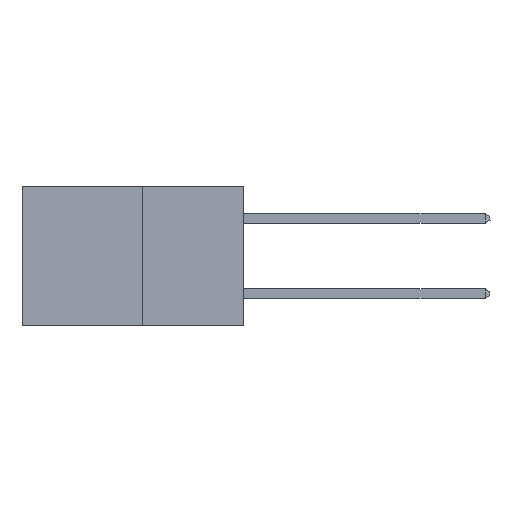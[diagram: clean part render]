
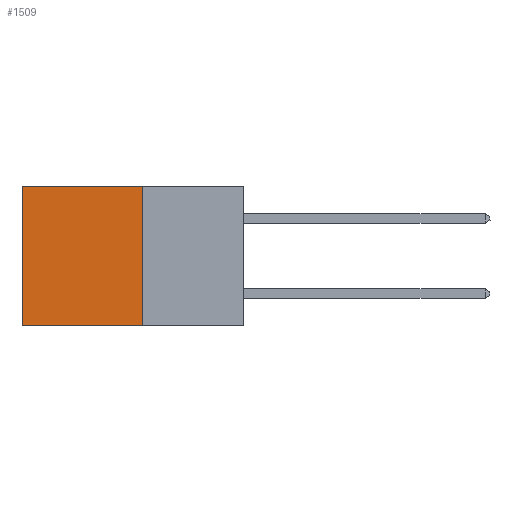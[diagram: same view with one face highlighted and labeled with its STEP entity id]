
A CAD part, left-side view. The second image highlights one B-rep face of the part: STEP entity #1509.
In plain terms, the highlighted planar face has unit normal (-1, 0, 0).
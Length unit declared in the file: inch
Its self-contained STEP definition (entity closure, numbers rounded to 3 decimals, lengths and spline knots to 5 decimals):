
#188 = ORIENTED_EDGE ( 'NONE', *, *, #4022, .T. ) ;
#232 = VERTEX_POINT ( 'NONE', #1717 ) ;
#594 = LINE ( 'NONE', #9998, #5398 ) ;
#685 = ORIENTED_EDGE ( 'NONE', *, *, #2946, .F. ) ;
#1406 = VERTEX_POINT ( 'NONE', #11083 ) ;
#1481 = AXIS2_PLACEMENT_3D ( 'NONE', #5484, #7393, #5969 ) ;
#1509 = ADVANCED_FACE ( 'NONE', ( #4404 ), #5711, .F. ) ;
#1717 = CARTESIAN_POINT ( 'NONE',  ( 0.277, 0.27, 0. ) ) ;
#2160 = EDGE_CURVE ( 'NONE', #1406, #3492, #8830, .T. ) ;
#2493 = EDGE_LOOP ( 'NONE', ( #188, #2841, #685, #4034 ) ) ;
#2841 = ORIENTED_EDGE ( 'NONE', *, *, #2160, .F. ) ;
#2946 = EDGE_CURVE ( 'NONE', #232, #1406, #10868, .T. ) ;
#3453 = VECTOR ( 'NONE', #9688, 39.37008 ) ;
#3492 = VERTEX_POINT ( 'NONE', #6788 ) ;
#4022 = EDGE_CURVE ( 'NONE', #5040, #3492, #594, .T. ) ;
#4034 = ORIENTED_EDGE ( 'NONE', *, *, #4761, .T. ) ;
#4404 = FACE_OUTER_BOUND ( 'NONE', #2493, .T. ) ;
#4761 = EDGE_CURVE ( 'NONE', #232, #5040, #9844, .T. ) ;
#5040 = VERTEX_POINT ( 'NONE', #11506 ) ;
#5154 = CARTESIAN_POINT ( 'NONE',  ( 0.277, 0.27, -0.37 ) ) ;
#5398 = VECTOR ( 'NONE', #9977, 39.37008 ) ;
#5484 = CARTESIAN_POINT ( 'NONE',  ( 0.277, 0.27, -0.37 ) ) ;
#5711 = PLANE ( 'NONE',  #1481 ) ;
#5969 = DIRECTION ( 'NONE',  ( 0., 0., -1. ) ) ;
#6788 = CARTESIAN_POINT ( 'NONE',  ( 0.277, 0.59, -0.37 ) ) ;
#7161 = DIRECTION ( 'NONE',  ( 0., 1., 0. ) ) ;
#7171 = CARTESIAN_POINT ( 'NONE',  ( 0.277, 0.27, 0. ) ) ;
#7393 = DIRECTION ( 'NONE',  ( 1., 0., 0. ) ) ;
#8791 = DIRECTION ( 'NONE',  ( 0., 0., -1. ) ) ;
#8806 = VECTOR ( 'NONE', #8791, 39.37008 ) ;
#8830 = LINE ( 'NONE', #5154, #3453 ) ;
#9688 = DIRECTION ( 'NONE',  ( 0., 1., 0. ) ) ;
#9844 = LINE ( 'NONE', #7171, #11463 ) ;
#9977 = DIRECTION ( 'NONE',  ( 0., 0., -1. ) ) ;
#9998 = CARTESIAN_POINT ( 'NONE',  ( 0.277, 0.59, -0.37 ) ) ;
#10868 = LINE ( 'NONE', #10938, #8806 ) ;
#10938 = CARTESIAN_POINT ( 'NONE',  ( 0.277, 0.27, -0.37 ) ) ;
#11083 = CARTESIAN_POINT ( 'NONE',  ( 0.277, 0.27, -0.37 ) ) ;
#11463 = VECTOR ( 'NONE', #7161, 39.37008 ) ;
#11506 = CARTESIAN_POINT ( 'NONE',  ( 0.277, 0.59, 0. ) ) ;
